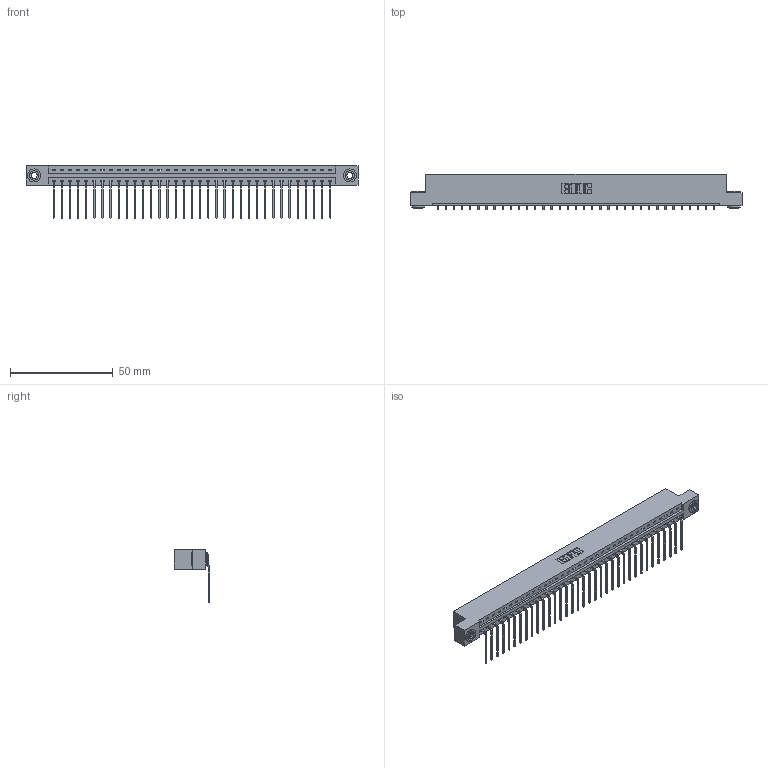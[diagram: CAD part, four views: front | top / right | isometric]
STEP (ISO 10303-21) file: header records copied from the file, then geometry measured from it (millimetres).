
FILE_DESCRIPTION (( 'STEP AP203' ), '1' );
FILE_NAME ('337-035-559-103.STEP', '2018-08-07T21:11:24', ( '' ), ( '' ), 'SwSTEP 2.0', 'SolidWorks 2016', '' );
FILE_SCHEMA (( 'CONFIG_CONTROL_DESIGN' ));
Length unit declared in the file: inch
Products named in the file (4): 345-250-002_345-250-002-102; 337-035-559-103; 337 Part_Flush Mounting Lugs - 0.156 Dia-TH; 345-292-001_558 559 Tail - 1
Assembly tree (38 placements, depth 2):
  337-035-559-103
    337 Part_Flush Mounting Lugs - 0.156 Dia-TH
    345-292-001_558 559 Tail - 1  x35
    345-250-002_345-250-002-102  x2
Bounding box: 161.7 x 17.09 x 25.53 mm (x, y, z)
Volume: 16854 mm3; surface area: 18326.4 mm2
Topology: 38 solids, 38 shells, 2392 faces, 7177 edges, 4734 vertices
Faces by surface type: plane 1760, cylinder 624, cone 8
Entity records: 27656 total; most frequent: CARTESIAN_POINT 4794, ORIENTED_EDGE 4758, DIRECTION 4083, EDGE_CURVE 2379, LINE 2227, VECTOR 2227, VERTEX_POINT 1582, AXIS2_PLACEMENT_3D 928
